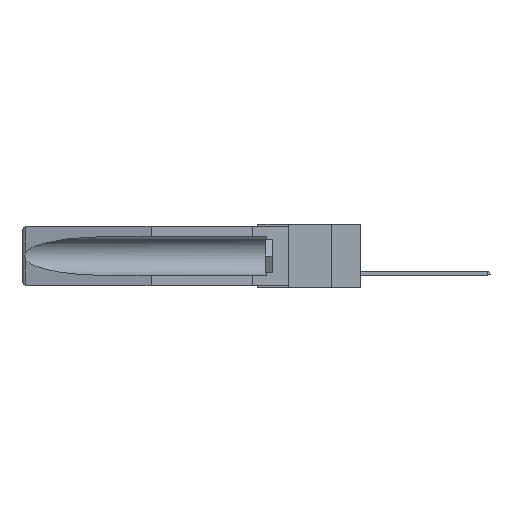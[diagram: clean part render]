
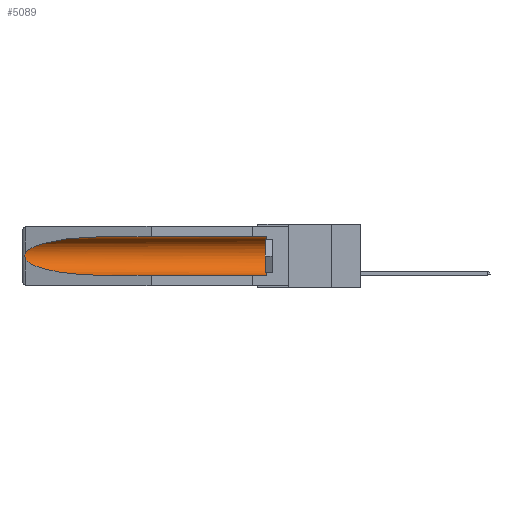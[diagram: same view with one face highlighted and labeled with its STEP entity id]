
A CAD part, left-side view. The second image highlights one B-rep face of the part: STEP entity #5089.
In plain terms, the highlighted cylindrical face has radius 2.857 mm (diameter 5.715 mm), a partial arc.
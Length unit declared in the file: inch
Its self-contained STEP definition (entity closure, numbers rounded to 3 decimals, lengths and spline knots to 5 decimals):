
#1020 = CARTESIAN_POINT ( 'NONE',  ( 0.21114, 1.30732, -0.059 ) ) ;
#1873 = CARTESIAN_POINT ( 'NONE',  ( 0.26537, 1.52718, -0.14972 ) ) ;
#1874 = CARTESIAN_POINT ( 'NONE',  ( 0.155, 0.126, -0.284 ) ) ;
#2568 = LINE ( 'NONE', #2815, #13020 ) ;
#2701 = B_SPLINE_CURVE_WITH_KNOTS ( 'NONE', 3,
 ( #1873, #10997, #4513, #24605, #8882, #19985, #15328, #26675, #6454, #4147 ),
 .UNSPECIFIED., .F., .F.,
 ( 4, 2, 2, 2, 4 ),
 ( 0., 0.00029, 0.00058, 0.00087, 0.00117 ),
 .UNSPECIFIED. ) ;
#2815 = CARTESIAN_POINT ( 'NONE',  ( 0.155, -0.30754, -0.059 ) ) ;
#3501 = CARTESIAN_POINT ( 'NONE',  ( 0.155, 1.07973, -0.059 ) ) ;
#4147 = CARTESIAN_POINT ( 'NONE',  ( 0.26537, 1.52718, -0.19328 ) ) ;
#4513 = CARTESIAN_POINT ( 'NONE',  ( 0.26654, 1.53092, -0.15636 ) ) ;
#5089 = ADVANCED_FACE ( 'NONE', ( #6653 ), #8837, .F. ) ;
#5420 = CARTESIAN_POINT ( 'NONE',  ( 0.155, 1.07973, -0.059 ) ) ;
#5662 = DIRECTION ( 'NONE',  ( 0., 1., 0. ) ) ;
#5860 = DIRECTION ( 'NONE',  ( 0., 0., 1. ) ) ;
#6454 = CARTESIAN_POINT ( 'NONE',  ( 0.26597, 1.5296, -0.19026 ) ) ;
#6653 = FACE_OUTER_BOUND ( 'NONE', #20836, .T. ) ;
#6683 = EDGE_CURVE ( 'NONE', #14815, #22236, #22919, .T. ) ;
#7753 = ORIENTED_EDGE ( 'NONE', *, *, #9761, .T. ) ;
#7963 = CARTESIAN_POINT ( 'NONE',  ( 0.26537, 1.52718, -0.14972 ) ) ;
#8725 = DIRECTION ( 'NONE',  ( 0., 1., 0. ) ) ;
#8837 = CYLINDRICAL_SURFACE ( 'NONE', #25045, 0.1125 ) ;
#8882 = CARTESIAN_POINT ( 'NONE',  ( 0.2675, 1.53308, -0.16763 ) ) ;
#9129 = ORIENTED_EDGE ( 'NONE', *, *, #6683, .T. ) ;
#9761 = EDGE_CURVE ( 'NONE', #22221, #17234, #21133, .T. ) ;
#9920 = VECTOR ( 'NONE', #5662, 39.37008 ) ;
#10456 = CARTESIAN_POINT ( 'NONE',  ( 0.155, -0.30754, -0.284 ) ) ;
#10589 = ORIENTED_EDGE ( 'NONE', *, *, #16650, .T. ) ;
#10699 = EDGE_CURVE ( 'NONE', #17234, #18456, #2568, .T. ) ;
#10822 = CARTESIAN_POINT ( 'NONE',  ( 0.26537, 1.52718, -0.19328 ) ) ;
#10997 = CARTESIAN_POINT ( 'NONE',  ( 0.26597, 1.52961, -0.15275 ) ) ;
#11721 = EDGE_CURVE ( 'NONE', #18456, #12509, #15221, .T. ) ;
#12509 = VERTEX_POINT ( 'NONE', #13035 ) ;
#12725 = DIRECTION ( 'NONE',  ( 0., 0., 1. ) ) ;
#13020 = VECTOR ( 'NONE', #14220, 39.37008 ) ;
#13035 = CARTESIAN_POINT ( 'NONE',  ( 0.26537, 1.52718, -0.14972 ) ) ;
#14220 = DIRECTION ( 'NONE',  ( 0., 1., 0. ) ) ;
#14444 = ORIENTED_EDGE ( 'NONE', *, *, #11721, .T. ) ;
#14675 = CARTESIAN_POINT ( 'NONE',  ( 0.155, 1.07973, -0.284 ) ) ;
#14815 = VERTEX_POINT ( 'NONE', #10822 ) ;
#15131 = CARTESIAN_POINT ( 'NONE',  ( 0.155, 1.07973, -0.284 ) ) ;
#15221 =( BOUNDED_CURVE ( )  B_SPLINE_CURVE ( 3, ( #5420, #1020, #28069, #7963 ),
 .UNSPECIFIED., .F., .F. ) 
 B_SPLINE_CURVE_WITH_KNOTS ( ( 4, 4 ),
 ( 4.71239, 6.08839 ),
 .UNSPECIFIED. ) 
 CURVE ( )  GEOMETRIC_REPRESENTATION_ITEM ( )  RATIONAL_B_SPLINE_CURVE ( ( 1., 0.848, 0.848, 1. ) ) 
 REPRESENTATION_ITEM ( '' )  );
#15328 = CARTESIAN_POINT ( 'NONE',  ( 0.2673, 1.53269, -0.17917 ) ) ;
#15560 = AXIS2_PLACEMENT_3D ( 'NONE', #19031, #19225, #5860 ) ;
#16650 = EDGE_CURVE ( 'NONE', #12509, #14815, #2701, .T. ) ;
#17234 = VERTEX_POINT ( 'NONE', #26365 ) ;
#18456 = VERTEX_POINT ( 'NONE', #3501 ) ;
#19031 = CARTESIAN_POINT ( 'NONE',  ( 0.155, 0.126, -0.1715 ) ) ;
#19225 = DIRECTION ( 'NONE',  ( 0., -1., 0. ) ) ;
#19506 = ORIENTED_EDGE ( 'NONE', *, *, #23319, .F. ) ;
#19854 = CARTESIAN_POINT ( 'NONE',  ( 0.155, -0.30754, -0.1715 ) ) ;
#19985 = CARTESIAN_POINT ( 'NONE',  ( 0.2675, 1.53308, -0.17534 ) ) ;
#20836 = EDGE_LOOP ( 'NONE', ( #14444, #10589, #9129, #19506, #7753, #22162 ) ) ;
#21133 = CIRCLE ( 'NONE', #15560, 0.1125 ) ;
#21612 = CARTESIAN_POINT ( 'NONE',  ( 0.25451, 1.48313, -0.24835 ) ) ;
#22162 = ORIENTED_EDGE ( 'NONE', *, *, #10699, .T. ) ;
#22221 = VERTEX_POINT ( 'NONE', #1874 ) ;
#22236 = VERTEX_POINT ( 'NONE', #15131 ) ;
#22919 =( BOUNDED_CURVE ( )  B_SPLINE_CURVE ( 3, ( #25855, #21612, #28063, #14675 ),
 .UNSPECIFIED., .F., .T. ) 
 B_SPLINE_CURVE_WITH_KNOTS ( ( 4, 4 ),
 ( 0.1948, 1.5708 ),
 .UNSPECIFIED. ) 
 CURVE ( )  GEOMETRIC_REPRESENTATION_ITEM ( )  RATIONAL_B_SPLINE_CURVE ( ( 1., 0.848, 0.848, 1. ) ) 
 REPRESENTATION_ITEM ( '' )  );
#23319 = EDGE_CURVE ( 'NONE', #22221, #22236, #23960, .T. ) ;
#23960 = LINE ( 'NONE', #10456, #9920 ) ;
#24605 = CARTESIAN_POINT ( 'NONE',  ( 0.2673, 1.5327, -0.16383 ) ) ;
#25045 = AXIS2_PLACEMENT_3D ( 'NONE', #19854, #8725, #12725 ) ;
#25855 = CARTESIAN_POINT ( 'NONE',  ( 0.26537, 1.52718, -0.19328 ) ) ;
#26365 = CARTESIAN_POINT ( 'NONE',  ( 0.155, 0.126, -0.059 ) ) ;
#26675 = CARTESIAN_POINT ( 'NONE',  ( 0.26655, 1.53094, -0.18657 ) ) ;
#28063 = CARTESIAN_POINT ( 'NONE',  ( 0.21114, 1.30732, -0.284 ) ) ;
#28069 = CARTESIAN_POINT ( 'NONE',  ( 0.25451, 1.48313, -0.09465 ) ) ;
